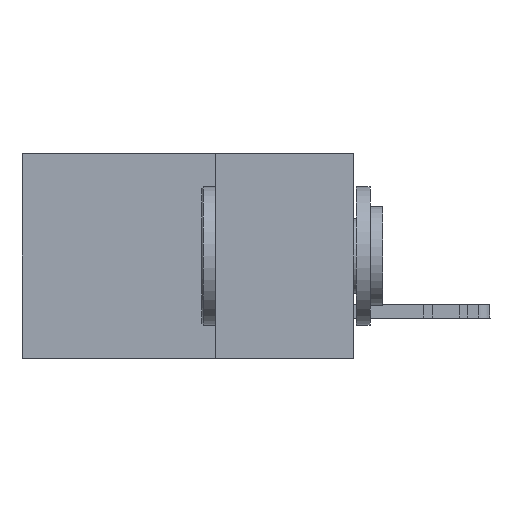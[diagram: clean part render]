
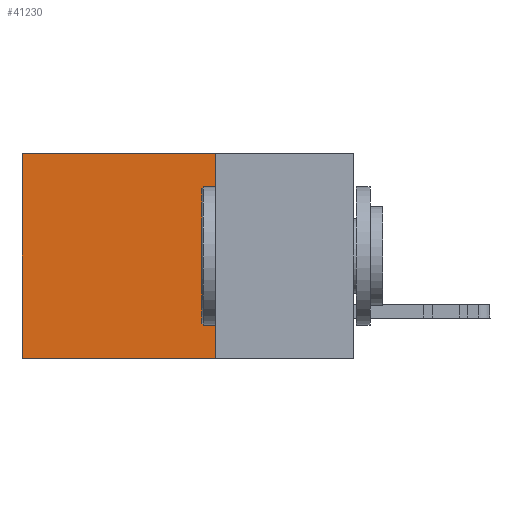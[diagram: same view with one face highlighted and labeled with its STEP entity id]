
A CAD part, left-side view. The second image highlights one B-rep face of the part: STEP entity #41230.
In plain terms, the highlighted planar face has unit normal (-1, 0, 0).
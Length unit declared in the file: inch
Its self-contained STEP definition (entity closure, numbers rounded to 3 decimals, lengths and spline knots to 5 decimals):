
#502 = VERTEX_POINT ( 'NONE', #14980 ) ;
#1056 = DIRECTION ( 'NONE',  ( 0., 1., 0. ) ) ;
#1633 = ORIENTED_EDGE ( 'NONE', *, *, #35645, .F. ) ;
#1839 = EDGE_LOOP ( 'NONE', ( #9279, #19476, #1633, #27396 ) ) ;
#4904 = LINE ( 'NONE', #15168, #25641 ) ;
#6015 = VERTEX_POINT ( 'NONE', #30635 ) ;
#6411 = VERTEX_POINT ( 'NONE', #17723 ) ;
#9279 = ORIENTED_EDGE ( 'NONE', *, *, #34703, .T. ) ;
#10509 = LINE ( 'NONE', #23317, #33415 ) ;
#10795 = VECTOR ( 'NONE', #11114, 39.37008 ) ;
#11114 = DIRECTION ( 'NONE',  ( 0., 1., 0. ) ) ;
#12400 = CARTESIAN_POINT ( 'NONE',  ( 0.2875, 0.25, 0. ) ) ;
#12710 = LINE ( 'NONE', #19201, #16997 ) ;
#14980 = CARTESIAN_POINT ( 'NONE',  ( 0.2875, 0.25, 0. ) ) ;
#15131 = FACE_OUTER_BOUND ( 'NONE', #1839, .T. ) ;
#15168 = CARTESIAN_POINT ( 'NONE',  ( 0.2875, 0.6, 0. ) ) ;
#16062 = DIRECTION ( 'NONE',  ( 0., 0., -1. ) ) ;
#16997 = VECTOR ( 'NONE', #16062, 39.37008 ) ;
#17723 = CARTESIAN_POINT ( 'NONE',  ( 0.2875, 0.25, -0.37 ) ) ;
#18379 = CARTESIAN_POINT ( 'NONE',  ( 0.2875, 0.25, 0. ) ) ;
#19201 = CARTESIAN_POINT ( 'NONE',  ( 0.2875, 0.25, 0. ) ) ;
#19476 = ORIENTED_EDGE ( 'NONE', *, *, #28385, .F. ) ;
#23264 = EDGE_CURVE ( 'NONE', #502, #33905, #30229, .T. ) ;
#23317 = CARTESIAN_POINT ( 'NONE',  ( 0.2875, 0.25, -0.37 ) ) ;
#25191 = DIRECTION ( 'NONE',  ( 0., 0., -1. ) ) ;
#25641 = VECTOR ( 'NONE', #36823, 39.37008 ) ;
#27396 = ORIENTED_EDGE ( 'NONE', *, *, #23264, .T. ) ;
#28153 = PLANE ( 'NONE',  #28528 ) ;
#28385 = EDGE_CURVE ( 'NONE', #6411, #6015, #10509, .T. ) ;
#28528 = AXIS2_PLACEMENT_3D ( 'NONE', #12400, #31095, #25191 ) ;
#30229 = LINE ( 'NONE', #18379, #10795 ) ;
#30635 = CARTESIAN_POINT ( 'NONE',  ( 0.2875, 0.6, -0.37 ) ) ;
#31095 = DIRECTION ( 'NONE',  ( 1., 0., 0. ) ) ;
#33415 = VECTOR ( 'NONE', #1056, 39.37008 ) ;
#33905 = VERTEX_POINT ( 'NONE', #33971 ) ;
#33971 = CARTESIAN_POINT ( 'NONE',  ( 0.2875, 0.6, 0. ) ) ;
#34703 = EDGE_CURVE ( 'NONE', #33905, #6015, #4904, .T. ) ;
#35645 = EDGE_CURVE ( 'NONE', #502, #6411, #12710, .T. ) ;
#36823 = DIRECTION ( 'NONE',  ( 0., 0., -1. ) ) ;
#41230 = ADVANCED_FACE ( 'NONE', ( #15131 ), #28153, .F. ) ;
